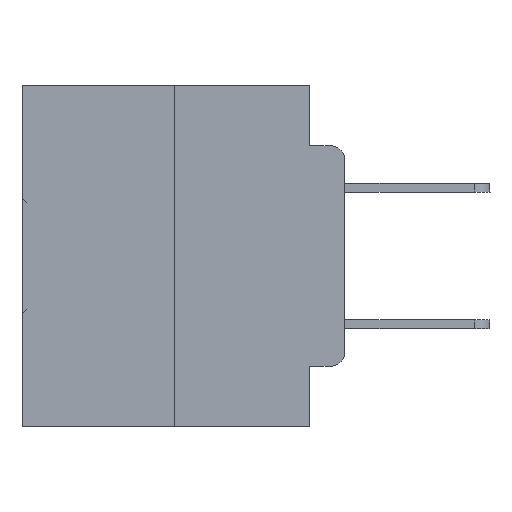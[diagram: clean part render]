
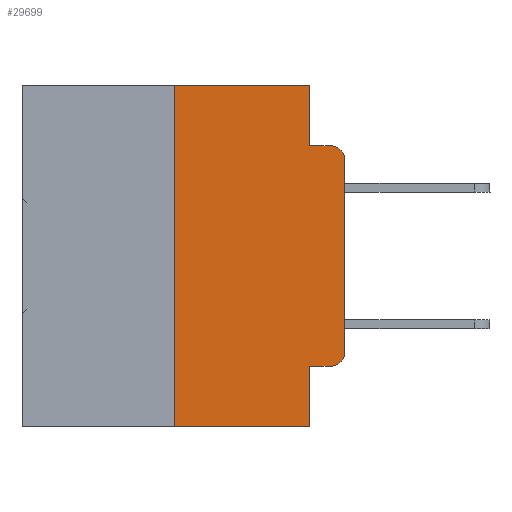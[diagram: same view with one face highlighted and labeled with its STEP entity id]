
A CAD part, left-side view. The second image highlights one B-rep face of the part: STEP entity #29699.
In plain terms, the highlighted planar face has unit normal (-1, 0, 0).
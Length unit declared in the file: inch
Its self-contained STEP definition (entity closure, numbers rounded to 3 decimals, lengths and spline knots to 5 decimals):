
#7 = DIRECTION ( 'NONE',  ( 0., 0., -1. ) ) ;
#100 = ORIENTED_EDGE ( 'NONE', *, *, #4020, .T. ) ;
#133 = EDGE_CURVE ( 'NONE', #29791, #9160, #18067, .T. ) ;
#471 = ORIENTED_EDGE ( 'NONE', *, *, #4970, .F. ) ;
#738 = CARTESIAN_POINT ( 'NONE',  ( 0., 0., -0.1085 ) ) ;
#814 = CARTESIAN_POINT ( 'NONE',  ( 0., 0.051, 0. ) ) ;
#978 = EDGE_CURVE ( 'NONE', #6980, #23256, #2666, .T. ) ;
#2323 = AXIS2_PLACEMENT_3D ( 'NONE', #17860, #23080, #20550 ) ;
#2666 = LINE ( 'NONE', #5352, #31186 ) ;
#2783 = CARTESIAN_POINT ( 'NONE',  ( 0., 0.051, -0.4115 ) ) ;
#2935 = EDGE_CURVE ( 'NONE', #26364, #31351, #32658, .T. ) ;
#2951 = DIRECTION ( 'NONE',  ( 0., 0., -1. ) ) ;
#3153 = EDGE_CURVE ( 'NONE', #23256, #31351, #31819, .T. ) ;
#4020 = EDGE_CURVE ( 'NONE', #9160, #6980, #18534, .T. ) ;
#4435 = CARTESIAN_POINT ( 'NONE',  ( 0., 0.051, -0.0885 ) ) ;
#4657 = EDGE_LOOP ( 'NONE', ( #12731, #24299, #24250, #23929, #28880, #471, #8253, #7822, #4907, #100 ) ) ;
#4873 = CARTESIAN_POINT ( 'NONE',  ( 0., 0.051, -0.4115 ) ) ;
#4907 = ORIENTED_EDGE ( 'NONE', *, *, #133, .T. ) ;
#4970 = EDGE_CURVE ( 'NONE', #16981, #21134, #22151, .T. ) ;
#5279 = EDGE_CURVE ( 'NONE', #16981, #22616, #28670, .T. ) ;
#5352 = CARTESIAN_POINT ( 'NONE',  ( 0., 0., 0. ) ) ;
#6638 = VECTOR ( 'NONE', #19568, 39.37008 ) ;
#6980 = VERTEX_POINT ( 'NONE', #14686 ) ;
#7822 = ORIENTED_EDGE ( 'NONE', *, *, #15966, .F. ) ;
#8041 = VERTEX_POINT ( 'NONE', #814 ) ;
#8253 = ORIENTED_EDGE ( 'NONE', *, *, #5279, .T. ) ;
#8354 = CARTESIAN_POINT ( 'NONE',  ( 0., 0.473, -0.5 ) ) ;
#8490 = CARTESIAN_POINT ( 'NONE',  ( 0., 0.051, 0. ) ) ;
#9160 = VERTEX_POINT ( 'NONE', #21526 ) ;
#9667 = VECTOR ( 'NONE', #7, 39.37008 ) ;
#9890 = EDGE_CURVE ( 'NONE', #8041, #26364, #13516, .T. ) ;
#10063 = VECTOR ( 'NONE', #2951, 39.37008 ) ;
#11527 = EDGE_CURVE ( 'NONE', #21134, #8041, #27777, .T. ) ;
#12583 = LINE ( 'NONE', #15430, #9667 ) ;
#12731 = ORIENTED_EDGE ( 'NONE', *, *, #978, .T. ) ;
#13516 = LINE ( 'NONE', #8490, #10063 ) ;
#14095 = DIRECTION ( 'NONE',  ( 0., 0., 1. ) ) ;
#14686 = CARTESIAN_POINT ( 'NONE',  ( 0., 0., -0.3915 ) ) ;
#15040 = CARTESIAN_POINT ( 'NONE',  ( 0., 0.25, 0. ) ) ;
#15107 = CARTESIAN_POINT ( 'NONE',  ( 0., 0.473, 0. ) ) ;
#15430 = CARTESIAN_POINT ( 'NONE',  ( 0., 0.051, 0. ) ) ;
#15434 = DIRECTION ( 'NONE',  ( -1., 0., 0. ) ) ;
#15966 = EDGE_CURVE ( 'NONE', #29791, #22616, #12583, .T. ) ;
#16981 = VERTEX_POINT ( 'NONE', #27206 ) ;
#17467 = PLANE ( 'NONE',  #31386 ) ;
#17860 = CARTESIAN_POINT ( 'NONE',  ( 0., 0.02, -0.1085 ) ) ;
#18067 = LINE ( 'NONE', #2783, #28982 ) ;
#18534 = CIRCLE ( 'NONE', #27631, 0.02 ) ;
#18606 = DIRECTION ( 'NONE',  ( 0., -1., 0. ) ) ;
#19177 = CARTESIAN_POINT ( 'NONE',  ( 0., 0.02, -0.0885 ) ) ;
#19568 = DIRECTION ( 'NONE',  ( 0., -1., 0. ) ) ;
#20550 = DIRECTION ( 'NONE',  ( 0., 0., -1. ) ) ;
#21117 = DIRECTION ( 'NONE',  ( 0., 0., 1. ) ) ;
#21134 = VERTEX_POINT ( 'NONE', #15040 ) ;
#21526 = CARTESIAN_POINT ( 'NONE',  ( 0., 0.02, -0.4115 ) ) ;
#22151 = LINE ( 'NONE', #31892, #32448 ) ;
#22576 = DIRECTION ( 'NONE',  ( 0., -1., 0. ) ) ;
#22616 = VERTEX_POINT ( 'NONE', #30376 ) ;
#23080 = DIRECTION ( 'NONE',  ( -1., 0., 0. ) ) ;
#23256 = VERTEX_POINT ( 'NONE', #738 ) ;
#23929 = ORIENTED_EDGE ( 'NONE', *, *, #9890, .F. ) ;
#24250 = ORIENTED_EDGE ( 'NONE', *, *, #2935, .F. ) ;
#24299 = ORIENTED_EDGE ( 'NONE', *, *, #3153, .T. ) ;
#25422 = CARTESIAN_POINT ( 'NONE',  ( 0., 0.473, 0. ) ) ;
#26364 = VERTEX_POINT ( 'NONE', #28685 ) ;
#27206 = CARTESIAN_POINT ( 'NONE',  ( 0., 0.25, -0.5 ) ) ;
#27534 = FACE_OUTER_BOUND ( 'NONE', #4657, .T. ) ;
#27631 = AXIS2_PLACEMENT_3D ( 'NONE', #30390, #15434, #30555 ) ;
#27709 = DIRECTION ( 'NONE',  ( 0., 0., -1. ) ) ;
#27777 = LINE ( 'NONE', #25422, #32090 ) ;
#28206 = DIRECTION ( 'NONE',  ( 1., 0., 0. ) ) ;
#28311 = DIRECTION ( 'NONE',  ( 0., -1., 0. ) ) ;
#28670 = LINE ( 'NONE', #8354, #31132 ) ;
#28685 = CARTESIAN_POINT ( 'NONE',  ( 0., 0.051, -0.0885 ) ) ;
#28880 = ORIENTED_EDGE ( 'NONE', *, *, #11527, .F. ) ;
#28982 = VECTOR ( 'NONE', #28311, 39.37008 ) ;
#29699 = ADVANCED_FACE ( 'NONE', ( #27534 ), #17467, .F. ) ;
#29791 = VERTEX_POINT ( 'NONE', #4873 ) ;
#30376 = CARTESIAN_POINT ( 'NONE',  ( 0., 0.051, -0.5 ) ) ;
#30390 = CARTESIAN_POINT ( 'NONE',  ( 0., 0.02, -0.3915 ) ) ;
#30555 = DIRECTION ( 'NONE',  ( 0., 0., -1. ) ) ;
#31132 = VECTOR ( 'NONE', #18606, 39.37008 ) ;
#31186 = VECTOR ( 'NONE', #21117, 39.37008 ) ;
#31351 = VERTEX_POINT ( 'NONE', #19177 ) ;
#31386 = AXIS2_PLACEMENT_3D ( 'NONE', #15107, #28206, #27709 ) ;
#31819 = CIRCLE ( 'NONE', #2323, 0.02 ) ;
#31892 = CARTESIAN_POINT ( 'NONE',  ( 0., 0.25, 0. ) ) ;
#32090 = VECTOR ( 'NONE', #22576, 39.37008 ) ;
#32448 = VECTOR ( 'NONE', #14095, 39.37008 ) ;
#32658 = LINE ( 'NONE', #4435, #6638 ) ;
